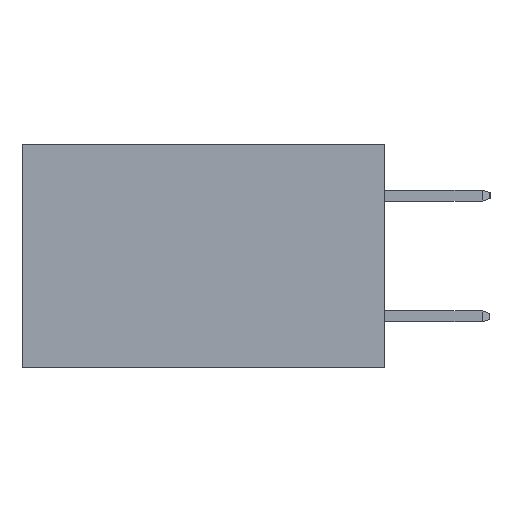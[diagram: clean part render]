
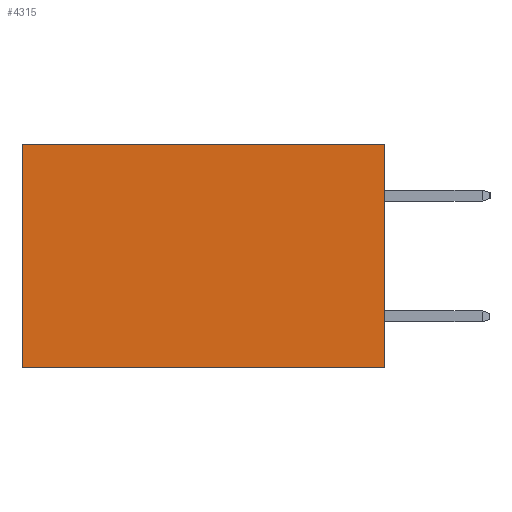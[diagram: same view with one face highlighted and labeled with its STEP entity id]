
A CAD part, left-side view. The second image highlights one B-rep face of the part: STEP entity #4315.
In plain terms, the highlighted planar face has unit normal (-1, 0, 0).
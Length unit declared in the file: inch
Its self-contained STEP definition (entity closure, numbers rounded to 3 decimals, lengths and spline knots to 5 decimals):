
#836 = CARTESIAN_POINT ( 'NONE',  ( 0.298, 0., 0. ) ) ;
#947 = CARTESIAN_POINT ( 'NONE',  ( 0.298, 0., -0.37 ) ) ;
#1611 = EDGE_CURVE ( 'NONE', #6289, #14894, #5407, .T. ) ;
#2353 = EDGE_CURVE ( 'NONE', #5862, #6289, #13675, .T. ) ;
#2648 = ORIENTED_EDGE ( 'NONE', *, *, #2353, .T. ) ;
#3163 = ORIENTED_EDGE ( 'NONE', *, *, #1611, .T. ) ;
#3180 = FACE_OUTER_BOUND ( 'NONE', #6482, .T. ) ;
#3706 = VERTEX_POINT ( 'NONE', #8560 ) ;
#3773 = VECTOR ( 'NONE', #12551, 39.37008 ) ;
#4315 = ADVANCED_FACE ( 'NONE', ( #3180 ), #7029, .F. ) ;
#5229 = EDGE_CURVE ( 'NONE', #5862, #3706, #12745, .T. ) ;
#5358 = DIRECTION ( 'NONE',  ( 0., 0., -1. ) ) ;
#5407 = LINE ( 'NONE', #7210, #5780 ) ;
#5780 = VECTOR ( 'NONE', #7182, 39.37008 ) ;
#5862 = VERTEX_POINT ( 'NONE', #6661 ) ;
#6289 = VERTEX_POINT ( 'NONE', #9004 ) ;
#6482 = EDGE_LOOP ( 'NONE', ( #3163, #7383, #8878, #2648 ) ) ;
#6661 = CARTESIAN_POINT ( 'NONE',  ( 0.298, 0., 0. ) ) ;
#6974 = DIRECTION ( 'NONE',  ( 1., 0., 0. ) ) ;
#7029 = PLANE ( 'NONE',  #7906 ) ;
#7182 = DIRECTION ( 'NONE',  ( 0., 0., -1. ) ) ;
#7210 = CARTESIAN_POINT ( 'NONE',  ( 0.298, 0.6, 0. ) ) ;
#7383 = ORIENTED_EDGE ( 'NONE', *, *, #14510, .F. ) ;
#7906 = AXIS2_PLACEMENT_3D ( 'NONE', #836, #6974, #5358 ) ;
#8560 = CARTESIAN_POINT ( 'NONE',  ( 0.298, 0., -0.37 ) ) ;
#8878 = ORIENTED_EDGE ( 'NONE', *, *, #5229, .F. ) ;
#9004 = CARTESIAN_POINT ( 'NONE',  ( 0.298, 0.6, 0. ) ) ;
#9702 = VECTOR ( 'NONE', #11571, 39.37008 ) ;
#11571 = DIRECTION ( 'NONE',  ( 0., 0., -1. ) ) ;
#12041 = CARTESIAN_POINT ( 'NONE',  ( 0.298, 0.6, -0.37 ) ) ;
#12236 = CARTESIAN_POINT ( 'NONE',  ( 0.298, 0., 0. ) ) ;
#12268 = DIRECTION ( 'NONE',  ( 0., 1., 0. ) ) ;
#12551 = DIRECTION ( 'NONE',  ( 0., 1., 0. ) ) ;
#12648 = LINE ( 'NONE', #947, #3773 ) ;
#12745 = LINE ( 'NONE', #13510, #9702 ) ;
#13332 = VECTOR ( 'NONE', #12268, 39.37008 ) ;
#13510 = CARTESIAN_POINT ( 'NONE',  ( 0.298, 0., 0. ) ) ;
#13675 = LINE ( 'NONE', #12236, #13332 ) ;
#14510 = EDGE_CURVE ( 'NONE', #3706, #14894, #12648, .T. ) ;
#14894 = VERTEX_POINT ( 'NONE', #12041 ) ;
